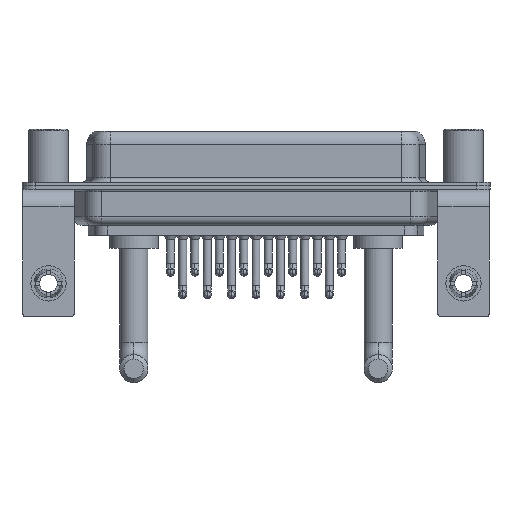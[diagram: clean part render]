
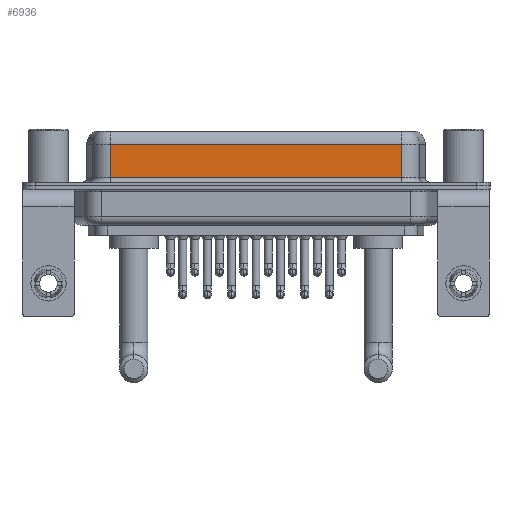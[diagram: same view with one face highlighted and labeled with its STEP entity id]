
A CAD part, front view. The second image highlights one B-rep face of the part: STEP entity #6936.
In plain terms, the highlighted planar face has unit normal (0, -1, 0).
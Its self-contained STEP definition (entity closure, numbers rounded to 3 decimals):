
#262 = CARTESIAN_POINT ( 'NONE',  ( 40.037, -3.95, 6.4 ) ) ;
#859 = DIRECTION ( 'NONE',  ( -1., 0., 0. ) ) ;
#942 = DIRECTION ( 'NONE',  ( 0., 0., 1. ) ) ;
#1194 = VERTEX_POINT ( 'NONE', #1359 ) ;
#1359 = CARTESIAN_POINT ( 'NONE',  ( 40.037, -3.95, 4.65 ) ) ;
#2202 = VECTOR ( 'NONE', #18759, 1000. ) ;
#2216 = EDGE_CURVE ( 'NONE', #1194, #9854, #20987, .T. ) ;
#2786 = FACE_OUTER_BOUND ( 'NONE', #21035, .T. ) ;
#2916 = CARTESIAN_POINT ( 'NONE',  ( 40.037, -3.95, 6.4 ) ) ;
#4120 = AXIS2_PLACEMENT_3D ( 'NONE', #2916, #17819, #942 ) ;
#4556 = VECTOR ( 'NONE', #15171, 1000. ) ;
#6656 = VERTEX_POINT ( 'NONE', #7378 ) ;
#6819 = CARTESIAN_POINT ( 'NONE',  ( 40.037, -3.95, 0.9 ) ) ;
#6936 = ADVANCED_FACE ( 'NONE', ( #2786 ), #10305, .F. ) ;
#7378 = CARTESIAN_POINT ( 'NONE',  ( 7.013, -3.95, 4.65 ) ) ;
#7451 = CARTESIAN_POINT ( 'NONE',  ( 40.037, -3.95, 0.9 ) ) ;
#8346 = EDGE_CURVE ( 'NONE', #1194, #6656, #14152, .T. ) ;
#8409 = ORIENTED_EDGE ( 'NONE', *, *, #8346, .T. ) ;
#8887 = ORIENTED_EDGE ( 'NONE', *, *, #2216, .F. ) ;
#9402 = CARTESIAN_POINT ( 'NONE',  ( 7.013, -3.95, 6.4 ) ) ;
#9444 = EDGE_CURVE ( 'NONE', #6656, #10878, #24238, .T. ) ;
#9527 = EDGE_CURVE ( 'NONE', #10878, #9854, #11367, .T. ) ;
#9854 = VERTEX_POINT ( 'NONE', #6819 ) ;
#10305 = PLANE ( 'NONE',  #4120 ) ;
#10878 = VERTEX_POINT ( 'NONE', #22592 ) ;
#11367 = LINE ( 'NONE', #7451, #4556 ) ;
#11593 = DIRECTION ( 'NONE',  ( 0., 0., -1. ) ) ;
#13855 = ORIENTED_EDGE ( 'NONE', *, *, #9527, .T. ) ;
#14030 = CARTESIAN_POINT ( 'NONE',  ( 40.037, -3.95, 4.65 ) ) ;
#14152 = LINE ( 'NONE', #14030, #17866 ) ;
#15171 = DIRECTION ( 'NONE',  ( 1., 0., 0. ) ) ;
#17040 = ORIENTED_EDGE ( 'NONE', *, *, #9444, .T. ) ;
#17819 = DIRECTION ( 'NONE',  ( 0., 1., 0. ) ) ;
#17866 = VECTOR ( 'NONE', #859, 1000. ) ;
#18759 = DIRECTION ( 'NONE',  ( 0., 0., -1. ) ) ;
#20987 = LINE ( 'NONE', #262, #23570 ) ;
#21035 = EDGE_LOOP ( 'NONE', ( #8887, #8409, #17040, #13855 ) ) ;
#22592 = CARTESIAN_POINT ( 'NONE',  ( 7.013, -3.95, 0.9 ) ) ;
#23570 = VECTOR ( 'NONE', #11593, 1000. ) ;
#24238 = LINE ( 'NONE', #9402, #2202 ) ;
